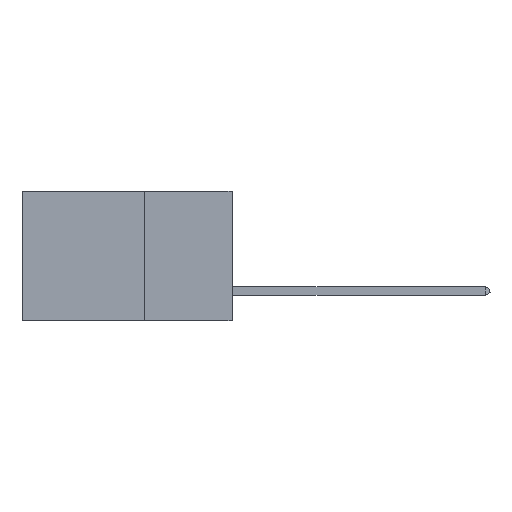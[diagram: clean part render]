
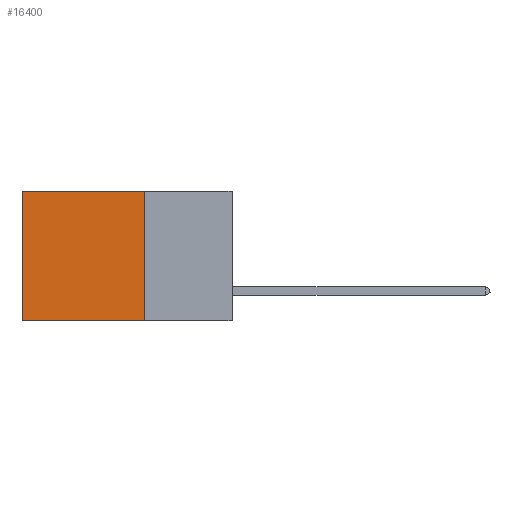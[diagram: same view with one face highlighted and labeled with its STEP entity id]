
A CAD part, left-side view. The second image highlights one B-rep face of the part: STEP entity #16400.
In plain terms, the highlighted planar face has unit normal (-1, 0, 0).
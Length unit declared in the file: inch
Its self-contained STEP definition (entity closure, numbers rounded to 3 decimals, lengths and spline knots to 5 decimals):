
#2245 = ORIENTED_EDGE ( 'NONE', *, *, #26724, .F. ) ;
#2821 = CARTESIAN_POINT ( 'NONE',  ( 0.2875, 0.25, -0.37 ) ) ;
#3251 = VECTOR ( 'NONE', #28896, 39.37008 ) ;
#5555 = VERTEX_POINT ( 'NONE', #2821 ) ;
#9905 = CARTESIAN_POINT ( 'NONE',  ( 0.2875, 0.25, 0. ) ) ;
#10164 = VERTEX_POINT ( 'NONE', #20497 ) ;
#12363 = EDGE_CURVE ( 'NONE', #24529, #16011, #32878, .T. ) ;
#12378 = CARTESIAN_POINT ( 'NONE',  ( 0.2875, 0.6, 0. ) ) ;
#16011 = VERTEX_POINT ( 'NONE', #18907 ) ;
#16383 = DIRECTION ( 'NONE',  ( 0., 0., -1. ) ) ;
#16400 = ADVANCED_FACE ( 'NONE', ( #17324 ), #27118, .F. ) ;
#17324 = FACE_OUTER_BOUND ( 'NONE', #35718, .T. ) ;
#18068 = ORIENTED_EDGE ( 'NONE', *, *, #28989, .F. ) ;
#18168 = CARTESIAN_POINT ( 'NONE',  ( 0.2875, 0.25, -0.37 ) ) ;
#18907 = CARTESIAN_POINT ( 'NONE',  ( 0.2875, 0.6, -0.37 ) ) ;
#20497 = CARTESIAN_POINT ( 'NONE',  ( 0.2875, 0.25, 0. ) ) ;
#22310 = CARTESIAN_POINT ( 'NONE',  ( 0.2875, 0.25, 0. ) ) ;
#22686 = VECTOR ( 'NONE', #26232, 39.37008 ) ;
#23411 = EDGE_CURVE ( 'NONE', #10164, #24529, #29547, .T. ) ;
#23571 = LINE ( 'NONE', #18168, #22686 ) ;
#24117 = DIRECTION ( 'NONE',  ( 0., 1., 0. ) ) ;
#24529 = VERTEX_POINT ( 'NONE', #12378 ) ;
#24859 = DIRECTION ( 'NONE',  ( 1., 0., 0. ) ) ;
#26232 = DIRECTION ( 'NONE',  ( 0., 1., 0. ) ) ;
#26724 = EDGE_CURVE ( 'NONE', #5555, #16011, #23571, .T. ) ;
#26954 = VECTOR ( 'NONE', #16383, 39.37008 ) ;
#27118 = PLANE ( 'NONE',  #31530 ) ;
#27276 = ORIENTED_EDGE ( 'NONE', *, *, #12363, .T. ) ;
#27722 = DIRECTION ( 'NONE',  ( 0., 0., -1. ) ) ;
#28896 = DIRECTION ( 'NONE',  ( 0., 0., -1. ) ) ;
#28989 = EDGE_CURVE ( 'NONE', #10164, #5555, #31376, .T. ) ;
#29547 = LINE ( 'NONE', #9905, #31743 ) ;
#31271 = CARTESIAN_POINT ( 'NONE',  ( 0.2875, 0.6, 0. ) ) ;
#31376 = LINE ( 'NONE', #22310, #26954 ) ;
#31530 = AXIS2_PLACEMENT_3D ( 'NONE', #33304, #24859, #27722 ) ;
#31679 = ORIENTED_EDGE ( 'NONE', *, *, #23411, .T. ) ;
#31743 = VECTOR ( 'NONE', #24117, 39.37008 ) ;
#32878 = LINE ( 'NONE', #31271, #3251 ) ;
#33304 = CARTESIAN_POINT ( 'NONE',  ( 0.2875, 0.25, 0. ) ) ;
#35718 = EDGE_LOOP ( 'NONE', ( #27276, #2245, #18068, #31679 ) ) ;
